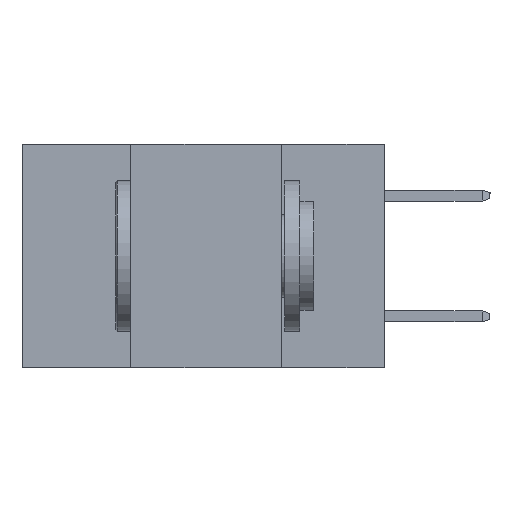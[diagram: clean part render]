
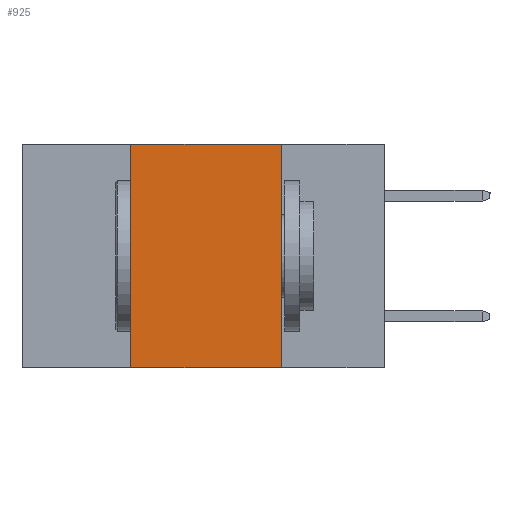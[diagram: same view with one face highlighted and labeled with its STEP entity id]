
A CAD part, left-side view. The second image highlights one B-rep face of the part: STEP entity #925.
In plain terms, the highlighted planar face has unit normal (-1, 0, 0).
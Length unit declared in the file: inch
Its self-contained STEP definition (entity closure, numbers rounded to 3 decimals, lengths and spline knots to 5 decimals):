
#183 = CARTESIAN_POINT ( 'NONE',  ( 0., 0.17, -0.37 ) ) ;
#925 = ADVANCED_FACE ( 'NONE', ( #1975 ), #7403, .F. ) ;
#1042 = ORIENTED_EDGE ( 'NONE', *, *, #4730, .F. ) ;
#1221 = EDGE_CURVE ( 'NONE', #1492, #5176, #5355, .T. ) ;
#1492 = VERTEX_POINT ( 'NONE', #7484 ) ;
#1560 = DIRECTION ( 'NONE',  ( 0., -1., 0. ) ) ;
#1631 = CARTESIAN_POINT ( 'NONE',  ( 0., 0.6, 0. ) ) ;
#1731 = VECTOR ( 'NONE', #2029, 39.37008 ) ;
#1871 = EDGE_CURVE ( 'NONE', #1492, #2463, #6308, .T. ) ;
#1975 = FACE_OUTER_BOUND ( 'NONE', #4080, .T. ) ;
#2029 = DIRECTION ( 'NONE',  ( 0., 0., -1. ) ) ;
#2240 = DIRECTION ( 'NONE',  ( 1., 0., 0. ) ) ;
#2463 = VERTEX_POINT ( 'NONE', #3308 ) ;
#3298 = LINE ( 'NONE', #10180, #9228 ) ;
#3308 = CARTESIAN_POINT ( 'NONE',  ( 0., 0.17, -0.37 ) ) ;
#3828 = VECTOR ( 'NONE', #10414, 39.37008 ) ;
#4080 = EDGE_LOOP ( 'NONE', ( #10458, #1042, #6663, #6382 ) ) ;
#4602 = VECTOR ( 'NONE', #1560, 39.37008 ) ;
#4730 = EDGE_CURVE ( 'NONE', #5176, #8731, #3298, .T. ) ;
#4838 = EDGE_CURVE ( 'NONE', #8731, #2463, #9637, .T. ) ;
#5176 = VERTEX_POINT ( 'NONE', #10890 ) ;
#5355 = LINE ( 'NONE', #8627, #3828 ) ;
#6308 = LINE ( 'NONE', #10807, #4602 ) ;
#6382 = ORIENTED_EDGE ( 'NONE', *, *, #1871, .T. ) ;
#6663 = ORIENTED_EDGE ( 'NONE', *, *, #1221, .F. ) ;
#7403 = PLANE ( 'NONE',  #7866 ) ;
#7484 = CARTESIAN_POINT ( 'NONE',  ( 0., 0.42, -0.37 ) ) ;
#7526 = DIRECTION ( 'NONE',  ( 0., -1., 0. ) ) ;
#7866 = AXIS2_PLACEMENT_3D ( 'NONE', #1631, #2240, #10876 ) ;
#8627 = CARTESIAN_POINT ( 'NONE',  ( 0., 0.42, -0.37 ) ) ;
#8731 = VERTEX_POINT ( 'NONE', #8745 ) ;
#8745 = CARTESIAN_POINT ( 'NONE',  ( 0., 0.17, 0. ) ) ;
#9228 = VECTOR ( 'NONE', #7526, 39.37008 ) ;
#9637 = LINE ( 'NONE', #183, #1731 ) ;
#10180 = CARTESIAN_POINT ( 'NONE',  ( 0., 0.6, 0. ) ) ;
#10414 = DIRECTION ( 'NONE',  ( 0., 0., 1. ) ) ;
#10458 = ORIENTED_EDGE ( 'NONE', *, *, #4838, .F. ) ;
#10807 = CARTESIAN_POINT ( 'NONE',  ( 0., 0.6, -0.37 ) ) ;
#10876 = DIRECTION ( 'NONE',  ( 0., 0., -1. ) ) ;
#10890 = CARTESIAN_POINT ( 'NONE',  ( 0., 0.42, 0. ) ) ;
